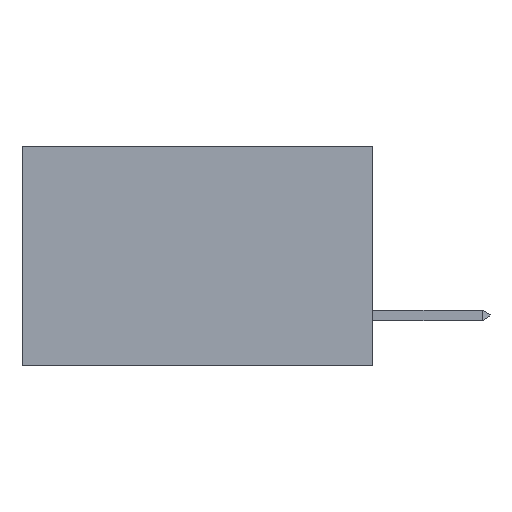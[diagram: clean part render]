
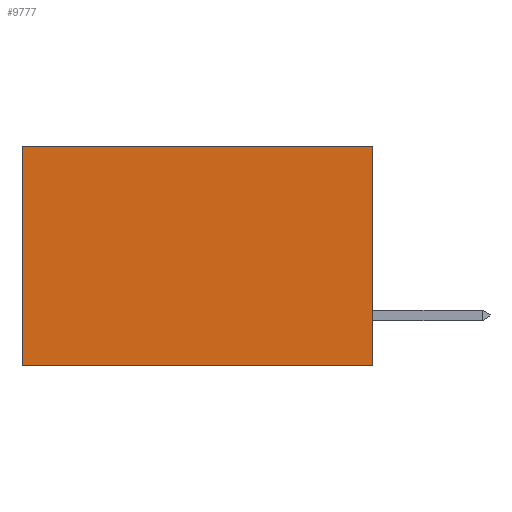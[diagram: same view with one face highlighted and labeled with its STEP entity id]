
A CAD part, left-side view. The second image highlights one B-rep face of the part: STEP entity #9777.
In plain terms, the highlighted planar face has unit normal (-1, 0, 0).
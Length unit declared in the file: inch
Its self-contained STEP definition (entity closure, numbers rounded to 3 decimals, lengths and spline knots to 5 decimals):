
#965 = LINE ( 'NONE', #3963, #9981 ) ;
#1771 = VERTEX_POINT ( 'NONE', #22250 ) ;
#3217 = EDGE_CURVE ( 'NONE', #1771, #24745, #4724, .T. ) ;
#3479 = VECTOR ( 'NONE', #17840, 39.37008 ) ;
#3940 = DIRECTION ( 'NONE',  ( 0., 1., 0. ) ) ;
#3963 = CARTESIAN_POINT ( 'NONE',  ( 0.277, 0., 0. ) ) ;
#4056 = LINE ( 'NONE', #19748, #3479 ) ;
#4558 = LINE ( 'NONE', #18437, #14320 ) ;
#4724 = LINE ( 'NONE', #13646, #5957 ) ;
#5957 = VECTOR ( 'NONE', #14400, 39.37008 ) ;
#6991 = CARTESIAN_POINT ( 'NONE',  ( 0.277, 0., 0. ) ) ;
#7918 = AXIS2_PLACEMENT_3D ( 'NONE', #17550, #17387, #17514 ) ;
#8217 = EDGE_CURVE ( 'NONE', #24740, #1771, #965, .T. ) ;
#9606 = FACE_OUTER_BOUND ( 'NONE', #20400, .T. ) ;
#9777 = ADVANCED_FACE ( 'NONE', ( #9606 ), #17687, .F. ) ;
#9981 = VECTOR ( 'NONE', #3940, 39.37008 ) ;
#10823 = VERTEX_POINT ( 'NONE', #19225 ) ;
#10882 = CARTESIAN_POINT ( 'NONE',  ( 0.277, 0.59, -0.37 ) ) ;
#10923 = ORIENTED_EDGE ( 'NONE', *, *, #13235, .F. ) ;
#11908 = ORIENTED_EDGE ( 'NONE', *, *, #3217, .T. ) ;
#13235 = EDGE_CURVE ( 'NONE', #24740, #10823, #4558, .T. ) ;
#13646 = CARTESIAN_POINT ( 'NONE',  ( 0.277, 0.59, -0.37 ) ) ;
#14320 = VECTOR ( 'NONE', #18193, 39.37008 ) ;
#14400 = DIRECTION ( 'NONE',  ( 0., 0., -1. ) ) ;
#17387 = DIRECTION ( 'NONE',  ( 1., 0., 0. ) ) ;
#17514 = DIRECTION ( 'NONE',  ( 0., 0., -1. ) ) ;
#17550 = CARTESIAN_POINT ( 'NONE',  ( 0.277, 0., -0.37 ) ) ;
#17687 = PLANE ( 'NONE',  #7918 ) ;
#17840 = DIRECTION ( 'NONE',  ( 0., 1., 0. ) ) ;
#18193 = DIRECTION ( 'NONE',  ( 0., 0., -1. ) ) ;
#18363 = ORIENTED_EDGE ( 'NONE', *, *, #19375, .F. ) ;
#18437 = CARTESIAN_POINT ( 'NONE',  ( 0.277, 0., -0.37 ) ) ;
#19225 = CARTESIAN_POINT ( 'NONE',  ( 0.277, 0., -0.37 ) ) ;
#19375 = EDGE_CURVE ( 'NONE', #10823, #24745, #4056, .T. ) ;
#19748 = CARTESIAN_POINT ( 'NONE',  ( 0.277, 0., -0.37 ) ) ;
#20125 = ORIENTED_EDGE ( 'NONE', *, *, #8217, .T. ) ;
#20400 = EDGE_LOOP ( 'NONE', ( #11908, #18363, #10923, #20125 ) ) ;
#22250 = CARTESIAN_POINT ( 'NONE',  ( 0.277, 0.59, 0. ) ) ;
#24740 = VERTEX_POINT ( 'NONE', #6991 ) ;
#24745 = VERTEX_POINT ( 'NONE', #10882 ) ;
